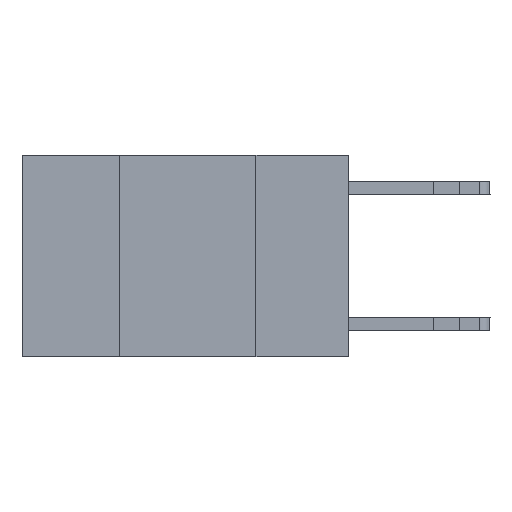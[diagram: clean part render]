
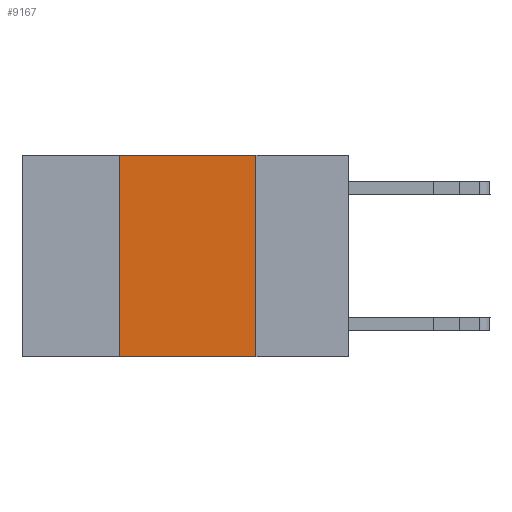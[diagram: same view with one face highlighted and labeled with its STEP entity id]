
A CAD part, left-side view. The second image highlights one B-rep face of the part: STEP entity #9167.
In plain terms, the highlighted planar face has unit normal (-1, 0, 0).
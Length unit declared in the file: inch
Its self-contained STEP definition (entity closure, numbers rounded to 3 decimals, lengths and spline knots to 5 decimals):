
#145 = EDGE_CURVE ( 'NONE', #5554, #15199, #19581, .T. ) ;
#188 = CARTESIAN_POINT ( 'NONE',  ( 0., 0.6, -0.37 ) ) ;
#582 = VECTOR ( 'NONE', #7027, 39.37008 ) ;
#825 = DIRECTION ( 'NONE',  ( 0., -1., 0. ) ) ;
#3114 = ORIENTED_EDGE ( 'NONE', *, *, #7734, .T. ) ;
#3343 = PLANE ( 'NONE',  #10527 ) ;
#3744 = DIRECTION ( 'NONE',  ( 1., 0., 0. ) ) ;
#5554 = VERTEX_POINT ( 'NONE', #6452 ) ;
#5663 = LINE ( 'NONE', #12187, #7713 ) ;
#6090 = CARTESIAN_POINT ( 'NONE',  ( 0., 0.17, 0. ) ) ;
#6452 = CARTESIAN_POINT ( 'NONE',  ( 0., 0.42, 0. ) ) ;
#6731 = EDGE_LOOP ( 'NONE', ( #14592, #6751, #14748, #3114 ) ) ;
#6751 = ORIENTED_EDGE ( 'NONE', *, *, #145, .F. ) ;
#7027 = DIRECTION ( 'NONE',  ( 0., 0., -1. ) ) ;
#7312 = VECTOR ( 'NONE', #825, 39.37008 ) ;
#7713 = VECTOR ( 'NONE', #12083, 39.37008 ) ;
#7734 = EDGE_CURVE ( 'NONE', #15807, #16733, #9633, .T. ) ;
#8623 = CARTESIAN_POINT ( 'NONE',  ( 0., 0.17, -0.37 ) ) ;
#9167 = ADVANCED_FACE ( 'NONE', ( #11077 ), #3343, .F. ) ;
#9633 = LINE ( 'NONE', #188, #14392 ) ;
#9939 = DIRECTION ( 'NONE',  ( 0., 0., -1. ) ) ;
#10084 = LINE ( 'NONE', #19989, #582 ) ;
#10527 = AXIS2_PLACEMENT_3D ( 'NONE', #17697, #3744, #9939 ) ;
#11077 = FACE_OUTER_BOUND ( 'NONE', #6731, .T. ) ;
#11173 = DIRECTION ( 'NONE',  ( 0., -1., 0. ) ) ;
#12083 = DIRECTION ( 'NONE',  ( 0., 0., 1. ) ) ;
#12187 = CARTESIAN_POINT ( 'NONE',  ( 0., 0.42, 0. ) ) ;
#13146 = CARTESIAN_POINT ( 'NONE',  ( 0., 0.6, 0. ) ) ;
#13452 = CARTESIAN_POINT ( 'NONE',  ( 0., 0.42, -0.37 ) ) ;
#14392 = VECTOR ( 'NONE', #11173, 39.37008 ) ;
#14592 = ORIENTED_EDGE ( 'NONE', *, *, #17618, .F. ) ;
#14748 = ORIENTED_EDGE ( 'NONE', *, *, #14812, .F. ) ;
#14812 = EDGE_CURVE ( 'NONE', #15807, #5554, #5663, .T. ) ;
#15199 = VERTEX_POINT ( 'NONE', #6090 ) ;
#15807 = VERTEX_POINT ( 'NONE', #13452 ) ;
#16733 = VERTEX_POINT ( 'NONE', #8623 ) ;
#17618 = EDGE_CURVE ( 'NONE', #15199, #16733, #10084, .T. ) ;
#17697 = CARTESIAN_POINT ( 'NONE',  ( 0., 0.6, 0. ) ) ;
#19581 = LINE ( 'NONE', #13146, #7312 ) ;
#19989 = CARTESIAN_POINT ( 'NONE',  ( 0., 0.17, 0. ) ) ;
